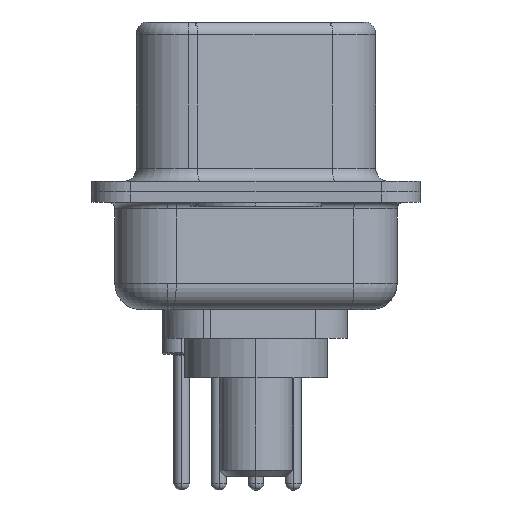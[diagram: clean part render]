
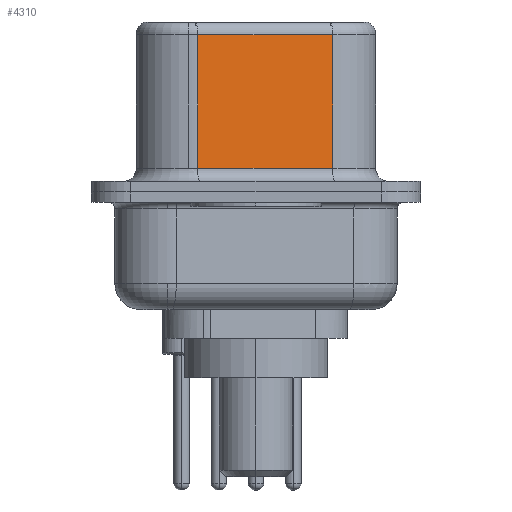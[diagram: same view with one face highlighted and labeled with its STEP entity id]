
A CAD part, left-side view. The second image highlights one B-rep face of the part: STEP entity #4310.
In plain terms, the highlighted planar face has unit normal (-0.985, -0.174, 0).
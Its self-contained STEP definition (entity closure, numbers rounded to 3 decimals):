
#761 = AXIS2_PLACEMENT_3D ( 'NONE', #6451, #16722, #12192 ) ;
#1322 = EDGE_CURVE ( 'NONE', #6598, #13238, #1552, .T. ) ;
#1552 = LINE ( 'NONE', #5187, #5257 ) ;
#1799 = EDGE_CURVE ( 'NONE', #6598, #8230, #2416, .T. ) ;
#2416 = LINE ( 'NONE', #11530, #13294 ) ;
#2859 = VECTOR ( 'NONE', #8633, 1000. ) ;
#4310 = ADVANCED_FACE ( 'NONE', ( #16636 ), #18271, .F. ) ;
#5187 = CARTESIAN_POINT ( 'NONE',  ( 4.58, -2.927, 6.52 ) ) ;
#5257 = VECTOR ( 'NONE', #11350, 1000. ) ;
#5785 = LINE ( 'NONE', #9426, #12953 ) ;
#6000 = EDGE_CURVE ( 'NONE', #16704, #13238, #5785, .T. ) ;
#6191 = LINE ( 'NONE', #17264, #2859 ) ;
#6451 = CARTESIAN_POINT ( 'NONE',  ( 4.58, -2.927, 6.52 ) ) ;
#6598 = VERTEX_POINT ( 'NONE', #13848 ) ;
#7160 = ORIENTED_EDGE ( 'NONE', *, *, #1799, .T. ) ;
#8230 = VERTEX_POINT ( 'NONE', #10459 ) ;
#8633 = DIRECTION ( 'NONE',  ( 0., 0., -1. ) ) ;
#9426 = CARTESIAN_POINT ( 'NONE',  ( 4.58, -2.927, 0.9 ) ) ;
#10459 = CARTESIAN_POINT ( 'NONE',  ( 3.67, 2.233, 6.02 ) ) ;
#11331 = EDGE_CURVE ( 'NONE', #8230, #16704, #6191, .T. ) ;
#11350 = DIRECTION ( 'NONE',  ( 0., 0., -1. ) ) ;
#11530 = CARTESIAN_POINT ( 'NONE',  ( 4.58, -2.927, 6.02 ) ) ;
#12185 = EDGE_LOOP ( 'NONE', ( #18457, #7160, #14407, #14115 ) ) ;
#12192 = DIRECTION ( 'NONE',  ( -0.174, 0.985, 0. ) ) ;
#12953 = VECTOR ( 'NONE', #15850, 1000. ) ;
#13238 = VERTEX_POINT ( 'NONE', #17867 ) ;
#13294 = VECTOR ( 'NONE', #14729, 1000. ) ;
#13848 = CARTESIAN_POINT ( 'NONE',  ( 4.58, -2.927, 6.02 ) ) ;
#14115 = ORIENTED_EDGE ( 'NONE', *, *, #6000, .T. ) ;
#14407 = ORIENTED_EDGE ( 'NONE', *, *, #11331, .T. ) ;
#14729 = DIRECTION ( 'NONE',  ( -0.174, 0.985, 0. ) ) ;
#15631 = CARTESIAN_POINT ( 'NONE',  ( 3.67, 2.233, 0.9 ) ) ;
#15850 = DIRECTION ( 'NONE',  ( 0.174, -0.985, 0. ) ) ;
#16636 = FACE_OUTER_BOUND ( 'NONE', #12185, .T. ) ;
#16704 = VERTEX_POINT ( 'NONE', #15631 ) ;
#16722 = DIRECTION ( 'NONE',  ( 0.985, 0.174, 0. ) ) ;
#17264 = CARTESIAN_POINT ( 'NONE',  ( 3.67, 2.233, 6.52 ) ) ;
#17867 = CARTESIAN_POINT ( 'NONE',  ( 4.58, -2.927, 0.9 ) ) ;
#18271 = PLANE ( 'NONE',  #761 ) ;
#18457 = ORIENTED_EDGE ( 'NONE', *, *, #1322, .F. ) ;
